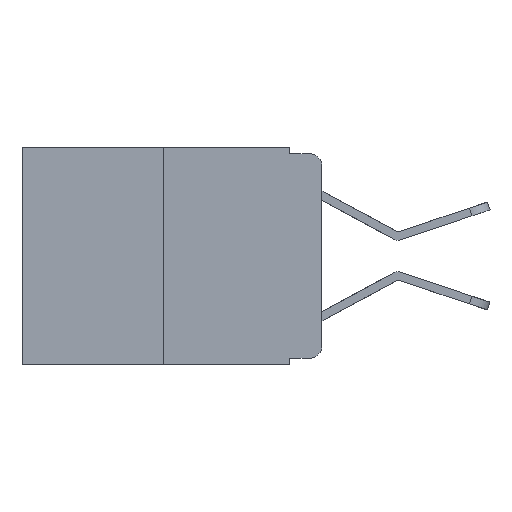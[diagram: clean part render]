
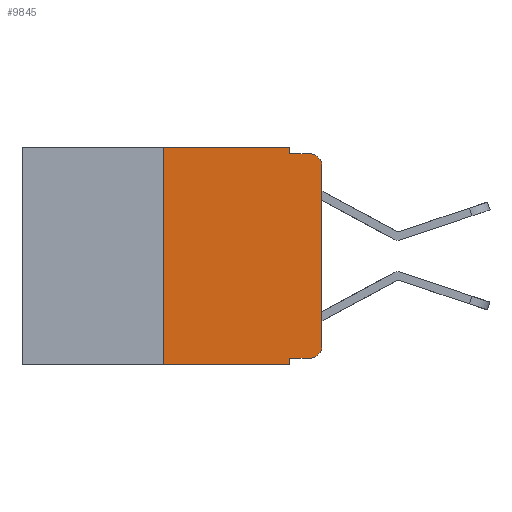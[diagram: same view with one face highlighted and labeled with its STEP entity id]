
A CAD part, left-side view. The second image highlights one B-rep face of the part: STEP entity #9845.
In plain terms, the highlighted planar face has unit normal (-1, 0, 0).
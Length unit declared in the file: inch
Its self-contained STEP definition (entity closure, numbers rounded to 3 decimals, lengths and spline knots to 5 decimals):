
#82 = DIRECTION ( 'NONE',  ( 0., -1., 0. ) ) ;
#346 = LINE ( 'NONE', #1961, #3078 ) ;
#465 = AXIS2_PLACEMENT_3D ( 'NONE', #2910, #7072, #2633 ) ;
#1201 = CARTESIAN_POINT ( 'NONE',  ( 0., 0., 0. ) ) ;
#1493 = VERTEX_POINT ( 'NONE', #6041 ) ;
#1511 = CARTESIAN_POINT ( 'NONE',  ( 0., 0.051, 0. ) ) ;
#1769 = CARTESIAN_POINT ( 'NONE',  ( 0., 0.02, -0.01 ) ) ;
#1932 = EDGE_CURVE ( 'NONE', #9081, #9958, #12668, .T. ) ;
#1941 = CIRCLE ( 'NONE', #14344, 0.02 ) ;
#1961 = CARTESIAN_POINT ( 'NONE',  ( 0., 0.051, -0.01 ) ) ;
#2069 = VERTEX_POINT ( 'NONE', #18629 ) ;
#2633 = DIRECTION ( 'NONE',  ( 0., 0., -1. ) ) ;
#2910 = CARTESIAN_POINT ( 'NONE',  ( 0., 0.02, -0.03 ) ) ;
#3078 = VECTOR ( 'NONE', #14748, 39.37008 ) ;
#3228 = EDGE_CURVE ( 'NONE', #11975, #2069, #18679, .T. ) ;
#3739 = CARTESIAN_POINT ( 'NONE',  ( 0., 0.25, 0. ) ) ;
#3790 = EDGE_LOOP ( 'NONE', ( #17196, #4752, #18523, #11777, #15966, #6585, #17044, #16212, #18563, #5784 ) ) ;
#4130 = DIRECTION ( 'NONE',  ( 0., 0., -1. ) ) ;
#4160 = FACE_OUTER_BOUND ( 'NONE', #3790, .T. ) ;
#4230 = CARTESIAN_POINT ( 'NONE',  ( 0., 0.051, -0.333 ) ) ;
#4294 = VECTOR ( 'NONE', #11053, 39.37008 ) ;
#4404 = LINE ( 'NONE', #11449, #6202 ) ;
#4752 = ORIENTED_EDGE ( 'NONE', *, *, #13552, .T. ) ;
#5483 = PLANE ( 'NONE',  #13041 ) ;
#5784 = ORIENTED_EDGE ( 'NONE', *, *, #7815, .T. ) ;
#6041 = CARTESIAN_POINT ( 'NONE',  ( 0., 0.051, -0.343 ) ) ;
#6202 = VECTOR ( 'NONE', #4130, 39.37008 ) ;
#6585 = ORIENTED_EDGE ( 'NONE', *, *, #1932, .F. ) ;
#6755 = VERTEX_POINT ( 'NONE', #1769 ) ;
#6817 = EDGE_CURVE ( 'NONE', #17979, #6755, #346, .T. ) ;
#6820 = CIRCLE ( 'NONE', #465, 0.02 ) ;
#7054 = CARTESIAN_POINT ( 'NONE',  ( 0., 0., -0.313 ) ) ;
#7072 = DIRECTION ( 'NONE',  ( -1., 0., 0. ) ) ;
#7594 = CARTESIAN_POINT ( 'NONE',  ( 0., 0.051, 0. ) ) ;
#7815 = EDGE_CURVE ( 'NONE', #2069, #14019, #1941, .T. ) ;
#7858 = CARTESIAN_POINT ( 'NONE',  ( 0., 0.02, -0.313 ) ) ;
#8147 = CARTESIAN_POINT ( 'NONE',  ( 0., 0.473, 0. ) ) ;
#8205 = CARTESIAN_POINT ( 'NONE',  ( 0., 0.051, -0.333 ) ) ;
#8551 = LINE ( 'NONE', #14347, #14544 ) ;
#9081 = VERTEX_POINT ( 'NONE', #15626 ) ;
#9497 = EDGE_CURVE ( 'NONE', #9958, #18404, #8551, .T. ) ;
#9845 = ADVANCED_FACE ( 'NONE', ( #4160 ), #5483, .F. ) ;
#9958 = VERTEX_POINT ( 'NONE', #13163 ) ;
#10191 = CARTESIAN_POINT ( 'NONE',  ( 0., 0.051, -0.01 ) ) ;
#10999 = DIRECTION ( 'NONE',  ( 0., 0., -1. ) ) ;
#11053 = DIRECTION ( 'NONE',  ( 0., 0., 1. ) ) ;
#11296 = DIRECTION ( 'NONE',  ( 1., 0., 0. ) ) ;
#11449 = CARTESIAN_POINT ( 'NONE',  ( 0., 0.051, 0. ) ) ;
#11546 = LINE ( 'NONE', #17438, #13482 ) ;
#11777 = ORIENTED_EDGE ( 'NONE', *, *, #17239, .F. ) ;
#11975 = VERTEX_POINT ( 'NONE', #8205 ) ;
#12186 = DIRECTION ( 'NONE',  ( 0., 0., 1. ) ) ;
#12232 = DIRECTION ( 'NONE',  ( -1., 0., 0. ) ) ;
#12474 = LINE ( 'NONE', #1201, #4294 ) ;
#12625 = DIRECTION ( 'NONE',  ( 0., -1., 0. ) ) ;
#12668 = LINE ( 'NONE', #3739, #14541 ) ;
#12691 = DIRECTION ( 'NONE',  ( 0., 0., -1. ) ) ;
#12708 = VECTOR ( 'NONE', #12862, 39.37008 ) ;
#12862 = DIRECTION ( 'NONE',  ( 0., 0., -1. ) ) ;
#12964 = CARTESIAN_POINT ( 'NONE',  ( 0., 0., -0.03 ) ) ;
#13041 = AXIS2_PLACEMENT_3D ( 'NONE', #8147, #11296, #12691 ) ;
#13163 = CARTESIAN_POINT ( 'NONE',  ( 0., 0.25, 0. ) ) ;
#13462 = EDGE_CURVE ( 'NONE', #9081, #1493, #11546, .T. ) ;
#13482 = VECTOR ( 'NONE', #82, 39.37008 ) ;
#13551 = EDGE_CURVE ( 'NONE', #11975, #1493, #4404, .T. ) ;
#13552 = EDGE_CURVE ( 'NONE', #17356, #6755, #6820, .T. ) ;
#14019 = VERTEX_POINT ( 'NONE', #7054 ) ;
#14344 = AXIS2_PLACEMENT_3D ( 'NONE', #7858, #12232, #10999 ) ;
#14347 = CARTESIAN_POINT ( 'NONE',  ( 0., 0.473, 0. ) ) ;
#14541 = VECTOR ( 'NONE', #12186, 39.37008 ) ;
#14544 = VECTOR ( 'NONE', #12625, 39.37008 ) ;
#14748 = DIRECTION ( 'NONE',  ( 0., -1., 0. ) ) ;
#15620 = VECTOR ( 'NONE', #17161, 39.37008 ) ;
#15626 = CARTESIAN_POINT ( 'NONE',  ( 0., 0.25, -0.343 ) ) ;
#15966 = ORIENTED_EDGE ( 'NONE', *, *, #9497, .F. ) ;
#16212 = ORIENTED_EDGE ( 'NONE', *, *, #13551, .F. ) ;
#16500 = EDGE_CURVE ( 'NONE', #14019, #17356, #12474, .T. ) ;
#17044 = ORIENTED_EDGE ( 'NONE', *, *, #13462, .T. ) ;
#17158 = LINE ( 'NONE', #1511, #12708 ) ;
#17161 = DIRECTION ( 'NONE',  ( 0., -1., 0. ) ) ;
#17196 = ORIENTED_EDGE ( 'NONE', *, *, #16500, .T. ) ;
#17239 = EDGE_CURVE ( 'NONE', #18404, #17979, #17158, .T. ) ;
#17356 = VERTEX_POINT ( 'NONE', #12964 ) ;
#17438 = CARTESIAN_POINT ( 'NONE',  ( 0., 0.473, -0.343 ) ) ;
#17979 = VERTEX_POINT ( 'NONE', #10191 ) ;
#18404 = VERTEX_POINT ( 'NONE', #7594 ) ;
#18523 = ORIENTED_EDGE ( 'NONE', *, *, #6817, .F. ) ;
#18563 = ORIENTED_EDGE ( 'NONE', *, *, #3228, .T. ) ;
#18629 = CARTESIAN_POINT ( 'NONE',  ( 0., 0.02, -0.333 ) ) ;
#18679 = LINE ( 'NONE', #4230, #15620 ) ;
